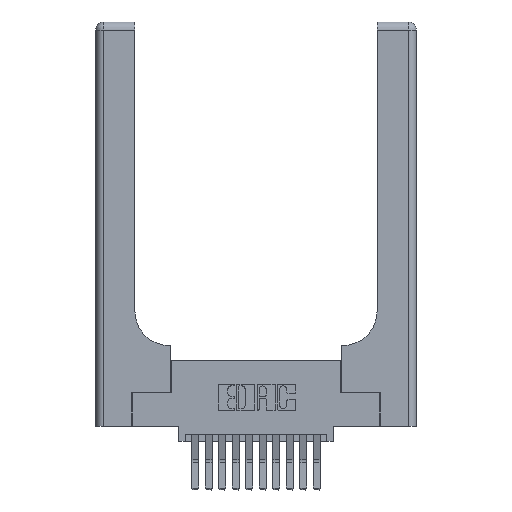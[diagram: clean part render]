
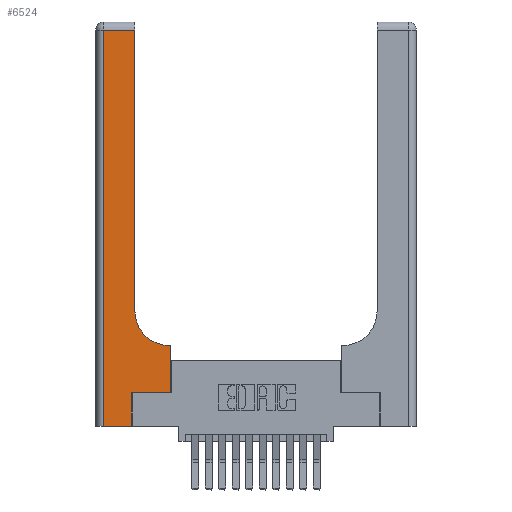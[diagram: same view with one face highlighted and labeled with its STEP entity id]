
A CAD part, top view. The second image highlights one B-rep face of the part: STEP entity #6524.
In plain terms, the highlighted planar face has unit normal (0, 0, 1).
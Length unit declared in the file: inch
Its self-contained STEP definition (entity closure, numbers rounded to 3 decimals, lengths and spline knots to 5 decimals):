
#165 = VECTOR ( 'NONE', #4046, 39.37008 ) ;
#607 = VERTEX_POINT ( 'NONE', #3786 ) ;
#624 = CARTESIAN_POINT ( 'NONE',  ( 0.269, 0., 0.37 ) ) ;
#872 = CARTESIAN_POINT ( 'NONE',  ( 0.06, 2.94, 0.37 ) ) ;
#1293 = AXIS2_PLACEMENT_3D ( 'NONE', #6565, #7907, #17395 ) ;
#1572 = ORIENTED_EDGE ( 'NONE', *, *, #7065, .T. ) ;
#1661 = VERTEX_POINT ( 'NONE', #872 ) ;
#1703 = VERTEX_POINT ( 'NONE', #14546 ) ;
#1822 = LINE ( 'NONE', #17001, #15766 ) ;
#2094 = VECTOR ( 'NONE', #11129, 39.37008 ) ;
#2130 = ORIENTED_EDGE ( 'NONE', *, *, #7668, .T. ) ;
#2387 = LINE ( 'NONE', #5333, #5561 ) ;
#2450 = VERTEX_POINT ( 'NONE', #16031 ) ;
#2698 = EDGE_CURVE ( 'NONE', #6724, #1703, #5321, .T. ) ;
#2937 = ORIENTED_EDGE ( 'NONE', *, *, #17257, .T. ) ;
#3483 = DIRECTION ( 'NONE',  ( 1., 0., 0. ) ) ;
#3786 = CARTESIAN_POINT ( 'NONE',  ( 0.269, 0.25, 0.37 ) ) ;
#4046 = DIRECTION ( 'NONE',  ( 0., 1., 0. ) ) ;
#4246 = CARTESIAN_POINT ( 'NONE',  ( 0.2915, 0.85, 0.37 ) ) ;
#4384 = CARTESIAN_POINT ( 'NONE',  ( 0.5585, 0.25, 0.37 ) ) ;
#5033 = CIRCLE ( 'NONE', #13310, 0.25 ) ;
#5114 = DIRECTION ( 'NONE',  ( 0., 0., -1. ) ) ;
#5242 = ORIENTED_EDGE ( 'NONE', *, *, #10608, .T. ) ;
#5321 = LINE ( 'NONE', #17432, #16124 ) ;
#5333 = CARTESIAN_POINT ( 'NONE',  ( 0., 2.94, 0.37 ) ) ;
#5561 = VECTOR ( 'NONE', #12072, 39.37008 ) ;
#6054 = VERTEX_POINT ( 'NONE', #11816 ) ;
#6124 = VECTOR ( 'NONE', #16040, 39.37008 ) ;
#6524 = ADVANCED_FACE ( 'NONE', ( #10984 ), #14693, .F. ) ;
#6565 = CARTESIAN_POINT ( 'NONE',  ( 0., 3., 0.37 ) ) ;
#6724 = VERTEX_POINT ( 'NONE', #4246 ) ;
#6734 = CARTESIAN_POINT ( 'NONE',  ( 0.269, 0., 0.37 ) ) ;
#7065 = EDGE_CURVE ( 'NONE', #12336, #607, #7369, .T. ) ;
#7224 = ORIENTED_EDGE ( 'NONE', *, *, #7465, .T. ) ;
#7369 = LINE ( 'NONE', #6734, #165 ) ;
#7465 = EDGE_CURVE ( 'NONE', #6054, #6724, #5033, .T. ) ;
#7668 = EDGE_CURVE ( 'NONE', #8625, #2450, #16055, .T. ) ;
#7907 = DIRECTION ( 'NONE',  ( 0., 0., -1. ) ) ;
#8112 = ORIENTED_EDGE ( 'NONE', *, *, #2698, .T. ) ;
#8625 = VERTEX_POINT ( 'NONE', #15788 ) ;
#10126 = LINE ( 'NONE', #14685, #6124 ) ;
#10285 = CARTESIAN_POINT ( 'NONE',  ( 0.06, 3., 0.37 ) ) ;
#10398 = CARTESIAN_POINT ( 'NONE',  ( 0.2915, 0.6, 0.37 ) ) ;
#10408 = VECTOR ( 'NONE', #17175, 39.37008 ) ;
#10590 = EDGE_CURVE ( 'NONE', #11606, #12336, #1822, .T. ) ;
#10608 = EDGE_CURVE ( 'NONE', #1661, #11606, #12163, .T. ) ;
#10984 = FACE_OUTER_BOUND ( 'NONE', #11974, .T. ) ;
#11129 = DIRECTION ( 'NONE',  ( 0., 1., 0. ) ) ;
#11606 = VERTEX_POINT ( 'NONE', #16389 ) ;
#11816 = CARTESIAN_POINT ( 'NONE',  ( 0.5415, 0.6, 0.37 ) ) ;
#11974 = EDGE_LOOP ( 'NONE', ( #8112, #12085, #5242, #15609, #1572, #2937, #2130, #17473, #7224 ) ) ;
#12072 = DIRECTION ( 'NONE',  ( -1., 0., 0. ) ) ;
#12085 = ORIENTED_EDGE ( 'NONE', *, *, #15613, .T. ) ;
#12163 = LINE ( 'NONE', #10285, #15341 ) ;
#12336 = VERTEX_POINT ( 'NONE', #624 ) ;
#12991 = DIRECTION ( 'NONE',  ( 0., -1., 0. ) ) ;
#13232 = CARTESIAN_POINT ( 'NONE',  ( 0.5415, 0.85, 0.37 ) ) ;
#13310 = AXIS2_PLACEMENT_3D ( 'NONE', #13232, #5114, #14594 ) ;
#14050 = LINE ( 'NONE', #10398, #10408 ) ;
#14546 = CARTESIAN_POINT ( 'NONE',  ( 0.2915, 2.94, 0.37 ) ) ;
#14594 = DIRECTION ( 'NONE',  ( 1., 0., 0. ) ) ;
#14685 = CARTESIAN_POINT ( 'NONE',  ( 0.269, 0.25, 0.37 ) ) ;
#14693 = PLANE ( 'NONE',  #1293 ) ;
#15064 = EDGE_CURVE ( 'NONE', #2450, #6054, #14050, .T. ) ;
#15341 = VECTOR ( 'NONE', #12991, 39.37008 ) ;
#15609 = ORIENTED_EDGE ( 'NONE', *, *, #10590, .T. ) ;
#15613 = EDGE_CURVE ( 'NONE', #1703, #1661, #2387, .T. ) ;
#15766 = VECTOR ( 'NONE', #3483, 39.37008 ) ;
#15788 = CARTESIAN_POINT ( 'NONE',  ( 0.5585, 0.25, 0.37 ) ) ;
#16031 = CARTESIAN_POINT ( 'NONE',  ( 0.5585, 0.6, 0.37 ) ) ;
#16040 = DIRECTION ( 'NONE',  ( 1., 0., 0. ) ) ;
#16055 = LINE ( 'NONE', #4384, #2094 ) ;
#16124 = VECTOR ( 'NONE', #17379, 39.37008 ) ;
#16389 = CARTESIAN_POINT ( 'NONE',  ( 0.06, 0., 0.37 ) ) ;
#17001 = CARTESIAN_POINT ( 'NONE',  ( 0., 0., 0.37 ) ) ;
#17175 = DIRECTION ( 'NONE',  ( -1., 0., 0. ) ) ;
#17257 = EDGE_CURVE ( 'NONE', #607, #8625, #10126, .T. ) ;
#17379 = DIRECTION ( 'NONE',  ( 0., 1., 0. ) ) ;
#17395 = DIRECTION ( 'NONE',  ( -1., 0., 0. ) ) ;
#17432 = CARTESIAN_POINT ( 'NONE',  ( 0.2915, 3., 0.37 ) ) ;
#17473 = ORIENTED_EDGE ( 'NONE', *, *, #15064, .T. ) ;
